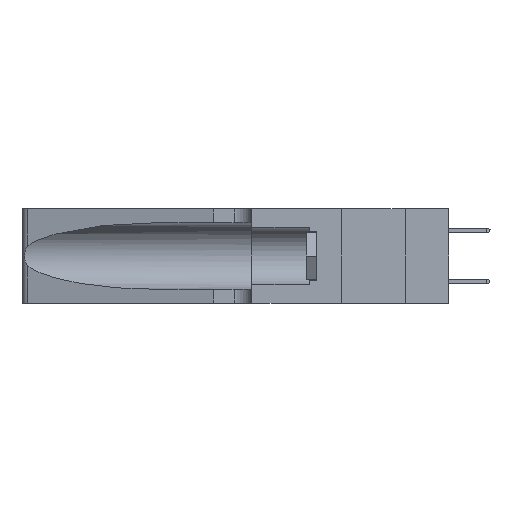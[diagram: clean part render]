
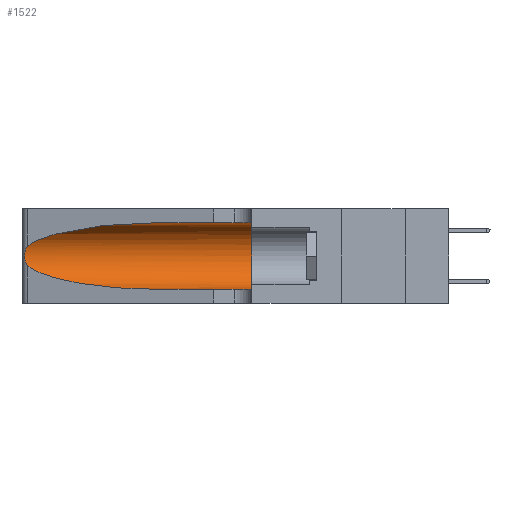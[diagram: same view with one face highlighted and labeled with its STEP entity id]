
A CAD part, left-side view. The second image highlights one B-rep face of the part: STEP entity #1522.
In plain terms, the highlighted cylindrical face has radius 3.308 mm (diameter 6.617 mm), a partial arc.
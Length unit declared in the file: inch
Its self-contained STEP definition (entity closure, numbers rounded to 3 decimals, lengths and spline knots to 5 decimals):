
#160 = CARTESIAN_POINT ( 'NONE',  ( 0.18966, 0.96281, 0.31525 ) ) ;
#204 = CARTESIAN_POINT ( 'NONE',  ( 0.1305, 1.61858, 0.31525 ) ) ;
#369 = FACE_OUTER_BOUND ( 'NONE', #35414, .T. ) ;
#782 = CARTESIAN_POINT ( 'NONE',  ( 0.2373, 1.15595, 0.28018 ) ) ;
#811 = CARTESIAN_POINT ( 'NONE',  ( 0.25856, 1.23593, 0.16098 ) ) ;
#1522 = ADVANCED_FACE ( 'NONE', ( #369 ), #8194, .F. ) ;
#2139 = ORIENTED_EDGE ( 'NONE', *, *, #34392, .T. ) ;
#2312 =( BOUNDED_CURVE ( )  B_SPLINE_CURVE ( 3, ( #15722, #160, #782, #25286 ),
 .UNSPECIFIED., .F., .T. ) 
 B_SPLINE_CURVE_WITH_KNOTS ( ( 4, 4 ),
 ( 1.5708, 2.84003 ),
 .UNSPECIFIED. ) 
 CURVE ( )  GEOMETRIC_REPRESENTATION_ITEM ( )  RATIONAL_B_SPLINE_CURVE ( ( 1., 0.87, 0.87, 1. ) ) 
 REPRESENTATION_ITEM ( '' )  );
#3628 = DIRECTION ( 'NONE',  ( 0., -1., 0. ) ) ;
#5821 = CARTESIAN_POINT ( 'NONE',  ( 0.1305, 0.35, 0.05475 ) ) ;
#6386 = CARTESIAN_POINT ( 'NONE',  ( 0.25789, 1.23486, 0.15765 ) ) ;
#6580 = LINE ( 'NONE', #17806, #10461 ) ;
#6639 = CARTESIAN_POINT ( 'NONE',  ( 0.25787, 1.23484, 0.2124 ) ) ;
#6791 = CARTESIAN_POINT ( 'NONE',  ( 0.1305, 1.61858, 0.185 ) ) ;
#6803 = EDGE_CURVE ( 'NONE', #23623, #15057, #6580, .T. ) ;
#6927 = EDGE_CURVE ( 'NONE', #29638, #15057, #34812, .T. ) ;
#7287 = VECTOR ( 'NONE', #13836, 39.37008 ) ;
#8194 = CYLINDRICAL_SURFACE ( 'NONE', #15801, 0.13025 ) ;
#9880 = VERTEX_POINT ( 'NONE', #28024 ) ;
#9917 = DIRECTION ( 'NONE',  ( 0., 1., 0. ) ) ;
#10078 = ORIENTED_EDGE ( 'NONE', *, *, #30514, .F. ) ;
#10215 = CARTESIAN_POINT ( 'NONE',  ( 0.1305, 0.35, 0.31525 ) ) ;
#10461 = VECTOR ( 'NONE', #3628, 39.37008 ) ;
#11148 = ORIENTED_EDGE ( 'NONE', *, *, #6803, .T. ) ;
#11734 = CARTESIAN_POINT ( 'NONE',  ( 0.26075, 1.23896, 0.178 ) ) ;
#12528 = B_SPLINE_CURVE_WITH_KNOTS ( 'NONE', 3,
 ( #25550, #22969, #20330, #6639, #31310, #22847, #28364, #11734, #28734, #811, #6386, #34332, #25776, #31170 ),
 .UNSPECIFIED., .F., .F.,
 ( 4, 2, 2, 2, 2, 2, 4 ),
 ( 0., 0.00027, 0.00053, 0.00107, 0.0016, 0.00187, 0.00214 ),
 .UNSPECIFIED. ) ;
#13836 = DIRECTION ( 'NONE',  ( 0., -1., 0. ) ) ;
#13847 = CARTESIAN_POINT ( 'NONE',  ( 0.25487, 1.22718, 0.14631 ) ) ;
#14117 = DIRECTION ( 'NONE',  ( 0., 0., -1. ) ) ;
#15057 = VERTEX_POINT ( 'NONE', #5821 ) ;
#15359 = DIRECTION ( 'NONE',  ( 0., 0., 1. ) ) ;
#15702 = ORIENTED_EDGE ( 'NONE', *, *, #17347, .T. ) ;
#15722 = CARTESIAN_POINT ( 'NONE',  ( 0.1305, 0.72297, 0.31525 ) ) ;
#15801 = AXIS2_PLACEMENT_3D ( 'NONE', #6791, #26197, #14117 ) ;
#16015 = CARTESIAN_POINT ( 'NONE',  ( 0.25487, 1.22718, 0.14631 ) ) ;
#16970 = CARTESIAN_POINT ( 'NONE',  ( 0.18966, 0.96281, 0.05475 ) ) ;
#17273 = EDGE_CURVE ( 'NONE', #20094, #9880, #2312, .T. ) ;
#17324 = CARTESIAN_POINT ( 'NONE',  ( 0.1305, 0.72297, 0.31525 ) ) ;
#17347 = EDGE_CURVE ( 'NONE', #9880, #23992, #12528, .T. ) ;
#17806 = CARTESIAN_POINT ( 'NONE',  ( 0.1305, 1.61858, 0.05475 ) ) ;
#18513 = CARTESIAN_POINT ( 'NONE',  ( 0.1305, 0.35, 0.185 ) ) ;
#20094 = VERTEX_POINT ( 'NONE', #17324 ) ;
#20330 = CARTESIAN_POINT ( 'NONE',  ( 0.25639, 1.23184, 0.21858 ) ) ;
#21831 = ORIENTED_EDGE ( 'NONE', *, *, #17273, .T. ) ;
#22847 = CARTESIAN_POINT ( 'NONE',  ( 0.26018, 1.23835, 0.19895 ) ) ;
#22969 = CARTESIAN_POINT ( 'NONE',  ( 0.25555, 1.22994, 0.2215 ) ) ;
#23623 = VERTEX_POINT ( 'NONE', #27699 ) ;
#23992 = VERTEX_POINT ( 'NONE', #16015 ) ;
#25098 = CARTESIAN_POINT ( 'NONE',  ( 0.1305, 0.72297, 0.05475 ) ) ;
#25286 = CARTESIAN_POINT ( 'NONE',  ( 0.25487, 1.22718, 0.22369 ) ) ;
#25550 = CARTESIAN_POINT ( 'NONE',  ( 0.25487, 1.22718, 0.22369 ) ) ;
#25776 = CARTESIAN_POINT ( 'NONE',  ( 0.25555, 1.22993, 0.14849 ) ) ;
#26197 = DIRECTION ( 'NONE',  ( 0., -1., 0. ) ) ;
#27676 = CARTESIAN_POINT ( 'NONE',  ( 0.2373, 1.15595, 0.08982 ) ) ;
#27699 = CARTESIAN_POINT ( 'NONE',  ( 0.1305, 0.72297, 0.05475 ) ) ;
#28024 = CARTESIAN_POINT ( 'NONE',  ( 0.25487, 1.22718, 0.22369 ) ) ;
#28364 = CARTESIAN_POINT ( 'NONE',  ( 0.26075, 1.23896, 0.19203 ) ) ;
#28734 = CARTESIAN_POINT ( 'NONE',  ( 0.26017, 1.23833, 0.17102 ) ) ;
#29244 =( BOUNDED_CURVE ( )  B_SPLINE_CURVE ( 3, ( #13847, #27676, #16970, #25098 ),
 .UNSPECIFIED., .F., .F. ) 
 B_SPLINE_CURVE_WITH_KNOTS ( ( 4, 4 ),
 ( 3.44316, 4.71239 ),
 .UNSPECIFIED. ) 
 CURVE ( )  GEOMETRIC_REPRESENTATION_ITEM ( )  RATIONAL_B_SPLINE_CURVE ( ( 1., 0.87, 0.87, 1. ) ) 
 REPRESENTATION_ITEM ( '' )  );
#29638 = VERTEX_POINT ( 'NONE', #10215 ) ;
#30215 = AXIS2_PLACEMENT_3D ( 'NONE', #18513, #9917, #15359 ) ;
#30368 = LINE ( 'NONE', #204, #7287 ) ;
#30514 = EDGE_CURVE ( 'NONE', #20094, #29638, #30368, .T. ) ;
#31170 = CARTESIAN_POINT ( 'NONE',  ( 0.25487, 1.22718, 0.14631 ) ) ;
#31310 = CARTESIAN_POINT ( 'NONE',  ( 0.25854, 1.2359, 0.20912 ) ) ;
#34332 = CARTESIAN_POINT ( 'NONE',  ( 0.25639, 1.23186, 0.15144 ) ) ;
#34392 = EDGE_CURVE ( 'NONE', #23992, #23623, #29244, .T. ) ;
#34656 = ORIENTED_EDGE ( 'NONE', *, *, #6927, .F. ) ;
#34812 = CIRCLE ( 'NONE', #30215, 0.13025 ) ;
#35414 = EDGE_LOOP ( 'NONE', ( #21831, #15702, #2139, #11148, #34656, #10078 ) ) ;
